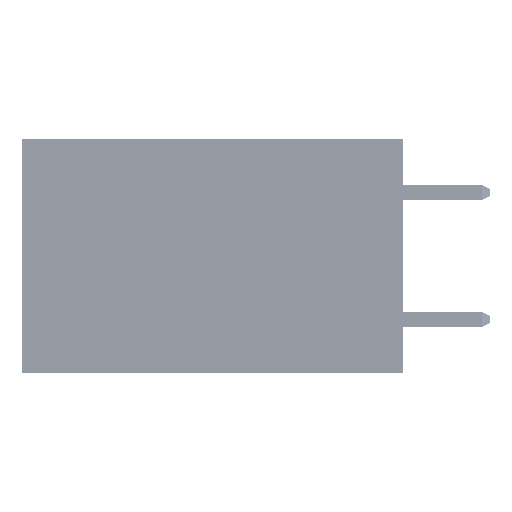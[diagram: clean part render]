
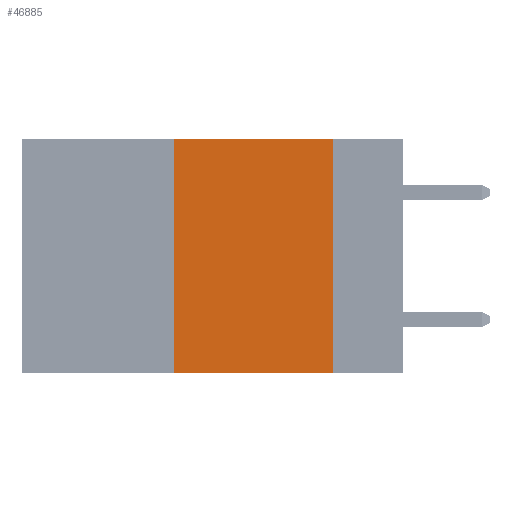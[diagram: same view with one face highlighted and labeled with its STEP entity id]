
A CAD part, left-side view. The second image highlights one B-rep face of the part: STEP entity #46885.
In plain terms, the highlighted planar face has unit normal (-1, 0, 0).
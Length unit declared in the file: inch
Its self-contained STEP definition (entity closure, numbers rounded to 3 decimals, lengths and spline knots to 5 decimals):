
#28 = EDGE_LOOP ( 'NONE', ( #29591, #30665, #38843, #5539 ) ) ;
#1971 = EDGE_CURVE ( 'NONE', #37790, #32000, #20864, .T. ) ;
#2121 = FACE_OUTER_BOUND ( 'NONE', #28, .T. ) ;
#2614 = LINE ( 'NONE', #25484, #13146 ) ;
#5539 = ORIENTED_EDGE ( 'NONE', *, *, #37696, .T. ) ;
#8023 = AXIS2_PLACEMENT_3D ( 'NONE', #17061, #47425, #39714 ) ;
#13146 = VECTOR ( 'NONE', #18029, 39.37008 ) ;
#15106 = CARTESIAN_POINT ( 'NONE',  ( 0., 0.36, 0. ) ) ;
#16403 = LINE ( 'NONE', #31576, #47940 ) ;
#17061 = CARTESIAN_POINT ( 'NONE',  ( 0., 0.6, 0. ) ) ;
#17367 = CARTESIAN_POINT ( 'NONE',  ( 0., 0.11, -0.37 ) ) ;
#18029 = DIRECTION ( 'NONE',  ( 0., 0., -1. ) ) ;
#20864 = LINE ( 'NONE', #21097, #23104 ) ;
#21097 = CARTESIAN_POINT ( 'NONE',  ( 0., 0.36, 0. ) ) ;
#21524 = EDGE_CURVE ( 'NONE', #35275, #22838, #2614, .T. ) ;
#21792 = CARTESIAN_POINT ( 'NONE',  ( 0., 0.6, 0. ) ) ;
#22838 = VERTEX_POINT ( 'NONE', #17367 ) ;
#23082 = CARTESIAN_POINT ( 'NONE',  ( 0., 0.11, 0. ) ) ;
#23104 = VECTOR ( 'NONE', #36042, 39.37008 ) ;
#24006 = EDGE_CURVE ( 'NONE', #32000, #35275, #33257, .T. ) ;
#24782 = DIRECTION ( 'NONE',  ( 0., -1., 0. ) ) ;
#25318 = CARTESIAN_POINT ( 'NONE',  ( 0., 0.36, -0.37 ) ) ;
#25484 = CARTESIAN_POINT ( 'NONE',  ( 0., 0.11, 0. ) ) ;
#29245 = VECTOR ( 'NONE', #24782, 39.37008 ) ;
#29591 = ORIENTED_EDGE ( 'NONE', *, *, #21524, .F. ) ;
#30665 = ORIENTED_EDGE ( 'NONE', *, *, #24006, .F. ) ;
#31576 = CARTESIAN_POINT ( 'NONE',  ( 0., 0.6, -0.37 ) ) ;
#32000 = VERTEX_POINT ( 'NONE', #15106 ) ;
#33257 = LINE ( 'NONE', #21792, #29245 ) ;
#35275 = VERTEX_POINT ( 'NONE', #23082 ) ;
#36042 = DIRECTION ( 'NONE',  ( 0., 0., 1. ) ) ;
#37696 = EDGE_CURVE ( 'NONE', #37790, #22838, #16403, .T. ) ;
#37790 = VERTEX_POINT ( 'NONE', #25318 ) ;
#38843 = ORIENTED_EDGE ( 'NONE', *, *, #1971, .F. ) ;
#39714 = DIRECTION ( 'NONE',  ( 0., 0., -1. ) ) ;
#39963 = PLANE ( 'NONE',  #8023 ) ;
#42536 = DIRECTION ( 'NONE',  ( 0., -1., 0. ) ) ;
#46885 = ADVANCED_FACE ( 'NONE', ( #2121 ), #39963, .F. ) ;
#47425 = DIRECTION ( 'NONE',  ( 1., 0., 0. ) ) ;
#47940 = VECTOR ( 'NONE', #42536, 39.37008 ) ;
